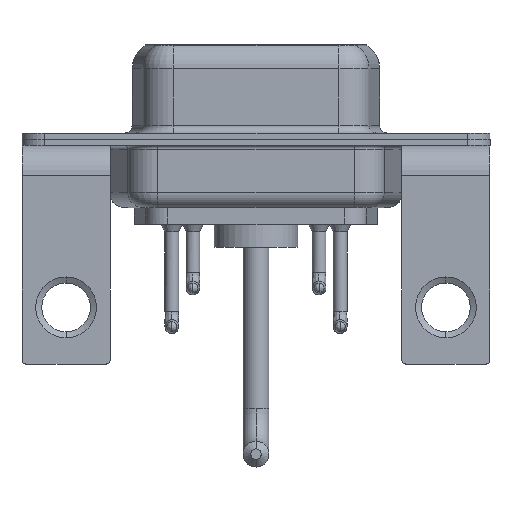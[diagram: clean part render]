
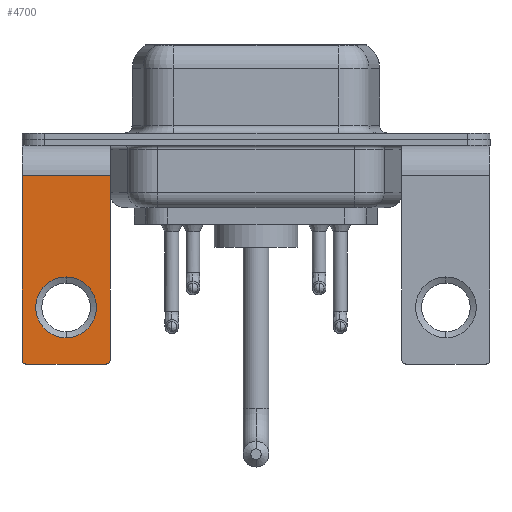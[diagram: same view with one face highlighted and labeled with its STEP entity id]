
A CAD part, front view. The second image highlights one B-rep face of the part: STEP entity #4700.
In plain terms, the highlighted planar face has unit normal (0, -1, 0).
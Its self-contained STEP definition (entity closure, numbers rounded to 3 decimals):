
#21 = EDGE_CURVE ( 'NONE', #16063, #6899, #4332, .T. ) ;
#58 = CIRCLE ( 'NONE', #14673, 2. ) ;
#65 = ORIENTED_EDGE ( 'NONE', *, *, #21, .T. ) ;
#187 = EDGE_CURVE ( 'NONE', #16063, #12076, #13276, .T. ) ;
#419 = ORIENTED_EDGE ( 'NONE', *, *, #11383, .T. ) ;
#754 = CARTESIAN_POINT ( 'NONE',  ( -2.9, -6.25, -2.4 ) ) ;
#839 = VERTEX_POINT ( 'NONE', #2353 ) ;
#1002 = VERTEX_POINT ( 'NONE', #13319 ) ;
#1269 = CARTESIAN_POINT ( 'NONE',  ( 2.65, -6.25, -14.55 ) ) ;
#1579 = VERTEX_POINT ( 'NONE', #5517 ) ;
#2065 = CIRCLE ( 'NONE', #7044, 2. ) ;
#2353 = CARTESIAN_POINT ( 'NONE',  ( 0., -6.25, -9.07 ) ) ;
#2690 = EDGE_CURVE ( 'NONE', #839, #9110, #58, .T. ) ;
#2698 = CARTESIAN_POINT ( 'NONE',  ( 2.65, -6.25, -14.8 ) ) ;
#2760 = FACE_BOUND ( 'NONE', #16592, .T. ) ;
#3486 = CARTESIAN_POINT ( 'NONE',  ( 2.9, -6.25, -2.4 ) ) ;
#3500 = AXIS2_PLACEMENT_3D ( 'NONE', #1269, #15760, #3951 ) ;
#3865 = DIRECTION ( 'NONE',  ( 0., 0., 1. ) ) ;
#3951 = DIRECTION ( 'NONE',  ( 0., 0., 1. ) ) ;
#4181 = DIRECTION ( 'NONE',  ( 0., 0., -1. ) ) ;
#4198 = CARTESIAN_POINT ( 'NONE',  ( 0., -6.25, -11.07 ) ) ;
#4213 = ORIENTED_EDGE ( 'NONE', *, *, #9050, .T. ) ;
#4332 = CIRCLE ( 'NONE', #3500, 0.25 ) ;
#4700 = ADVANCED_FACE ( 'NONE', ( #2760, #13208 ), #4892, .F. ) ;
#4892 = PLANE ( 'NONE',  #7012 ) ;
#4913 = VERTEX_POINT ( 'NONE', #754 ) ;
#5357 = CARTESIAN_POINT ( 'NONE',  ( 2.9, -6.25, -2.4 ) ) ;
#5517 = CARTESIAN_POINT ( 'NONE',  ( 2.9, -6.25, -2.4 ) ) ;
#5688 = CARTESIAN_POINT ( 'NONE',  ( -2.9, -6.25, -2.4 ) ) ;
#6351 = VECTOR ( 'NONE', #4181, 1000. ) ;
#6658 = CARTESIAN_POINT ( 'NONE',  ( 0., -6.25, -11.07 ) ) ;
#6764 = AXIS2_PLACEMENT_3D ( 'NONE', #11741, #9398, #13381 ) ;
#6899 = VERTEX_POINT ( 'NONE', #14375 ) ;
#6991 = ORIENTED_EDGE ( 'NONE', *, *, #187, .F. ) ;
#7012 = AXIS2_PLACEMENT_3D ( 'NONE', #5357, #8031, #11912 ) ;
#7044 = AXIS2_PLACEMENT_3D ( 'NONE', #4198, #14306, #3865 ) ;
#7105 = VECTOR ( 'NONE', #9968, 1000. ) ;
#7236 = CARTESIAN_POINT ( 'NONE',  ( 0., -6.25, -13.07 ) ) ;
#7364 = DIRECTION ( 'NONE',  ( -1., 0., 0. ) ) ;
#7646 = VECTOR ( 'NONE', #7364, 1000. ) ;
#8031 = DIRECTION ( 'NONE',  ( 0., 1., 0. ) ) ;
#8117 = DIRECTION ( 'NONE',  ( 0., 0., 1. ) ) ;
#9050 = EDGE_CURVE ( 'NONE', #1002, #12076, #13920, .T. ) ;
#9110 = VERTEX_POINT ( 'NONE', #7236 ) ;
#9398 = DIRECTION ( 'NONE',  ( 0., -1., 0. ) ) ;
#9416 = EDGE_CURVE ( 'NONE', #9110, #839, #2065, .T. ) ;
#9636 = LINE ( 'NONE', #5688, #7105 ) ;
#9949 = LINE ( 'NONE', #3486, #7646 ) ;
#9965 = CARTESIAN_POINT ( 'NONE',  ( 2.9, -6.25, -14.8 ) ) ;
#9968 = DIRECTION ( 'NONE',  ( 0., 0., -1. ) ) ;
#10738 = LINE ( 'NONE', #14538, #6351 ) ;
#11383 = EDGE_CURVE ( 'NONE', #4913, #1002, #9636, .T. ) ;
#11535 = VECTOR ( 'NONE', #13784, 1000. ) ;
#11673 = ORIENTED_EDGE ( 'NONE', *, *, #14144, .F. ) ;
#11741 = CARTESIAN_POINT ( 'NONE',  ( -2.65, -6.25, -14.55 ) ) ;
#11828 = ORIENTED_EDGE ( 'NONE', *, *, #2690, .T. ) ;
#11912 = DIRECTION ( 'NONE',  ( 0., 0., 1. ) ) ;
#11993 = EDGE_CURVE ( 'NONE', #1579, #4913, #9949, .T. ) ;
#12076 = VERTEX_POINT ( 'NONE', #14186 ) ;
#13208 = FACE_OUTER_BOUND ( 'NONE', #13222, .T. ) ;
#13222 = EDGE_LOOP ( 'NONE', ( #419, #4213, #6991, #65, #11673, #14833 ) ) ;
#13276 = LINE ( 'NONE', #9965, #11535 ) ;
#13319 = CARTESIAN_POINT ( 'NONE',  ( -2.9, -6.25, -14.55 ) ) ;
#13381 = DIRECTION ( 'NONE',  ( 0., 0., 1. ) ) ;
#13784 = DIRECTION ( 'NONE',  ( -1., 0., 0. ) ) ;
#13920 = CIRCLE ( 'NONE', #6764, 0.25 ) ;
#14144 = EDGE_CURVE ( 'NONE', #1579, #6899, #10738, .T. ) ;
#14186 = CARTESIAN_POINT ( 'NONE',  ( -2.65, -6.25, -14.8 ) ) ;
#14306 = DIRECTION ( 'NONE',  ( 0., 1., 0. ) ) ;
#14349 = ORIENTED_EDGE ( 'NONE', *, *, #9416, .T. ) ;
#14375 = CARTESIAN_POINT ( 'NONE',  ( 2.9, -6.25, -14.55 ) ) ;
#14538 = CARTESIAN_POINT ( 'NONE',  ( 2.9, -6.25, -2.4 ) ) ;
#14673 = AXIS2_PLACEMENT_3D ( 'NONE', #6658, #15874, #8117 ) ;
#14833 = ORIENTED_EDGE ( 'NONE', *, *, #11993, .T. ) ;
#15760 = DIRECTION ( 'NONE',  ( 0., -1., 0. ) ) ;
#15874 = DIRECTION ( 'NONE',  ( 0., 1., 0. ) ) ;
#16063 = VERTEX_POINT ( 'NONE', #2698 ) ;
#16592 = EDGE_LOOP ( 'NONE', ( #14349, #11828 ) ) ;
